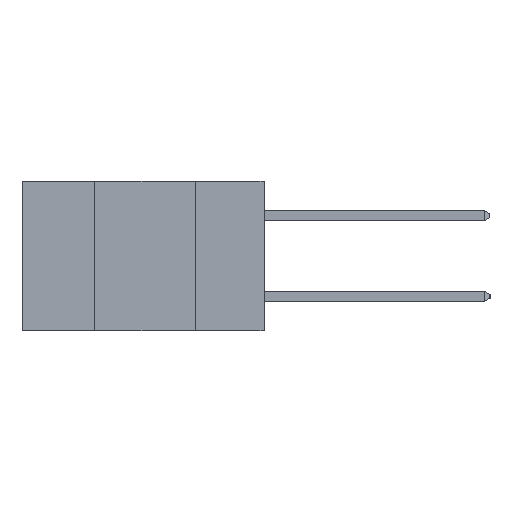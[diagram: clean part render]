
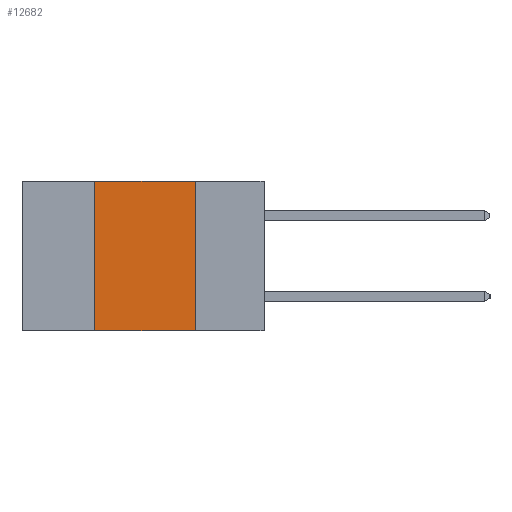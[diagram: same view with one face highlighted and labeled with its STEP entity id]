
A CAD part, left-side view. The second image highlights one B-rep face of the part: STEP entity #12682.
In plain terms, the highlighted planar face has unit normal (-1, 0, 0).
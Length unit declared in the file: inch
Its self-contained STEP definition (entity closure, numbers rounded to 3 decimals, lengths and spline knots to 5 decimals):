
#1041 = EDGE_CURVE ( 'NONE', #14348, #5909, #7604, .T. ) ;
#1482 = EDGE_LOOP ( 'NONE', ( #12746, #18399, #15497, #16934 ) ) ;
#1537 = VERTEX_POINT ( 'NONE', #18172 ) ;
#2102 = DIRECTION ( 'NONE',  ( 0., 0., -1. ) ) ;
#2430 = LINE ( 'NONE', #8013, #11968 ) ;
#3101 = DIRECTION ( 'NONE',  ( 0., -1., 0. ) ) ;
#3197 = DIRECTION ( 'NONE',  ( 0., -1., 0. ) ) ;
#4484 = VECTOR ( 'NONE', #3101, 39.37008 ) ;
#5244 = PLANE ( 'NONE',  #9983 ) ;
#5909 = VERTEX_POINT ( 'NONE', #8894 ) ;
#6665 = FACE_OUTER_BOUND ( 'NONE', #1482, .T. ) ;
#6901 = CARTESIAN_POINT ( 'NONE',  ( 0., 0.42, -0.37 ) ) ;
#7604 = LINE ( 'NONE', #6901, #19320 ) ;
#8013 = CARTESIAN_POINT ( 'NONE',  ( 0., 0.6, -0.37 ) ) ;
#8799 = DIRECTION ( 'NONE',  ( 0., 0., -1. ) ) ;
#8894 = CARTESIAN_POINT ( 'NONE',  ( 0., 0.42, 0. ) ) ;
#9983 = AXIS2_PLACEMENT_3D ( 'NONE', #10074, #11709, #2102 ) ;
#10074 = CARTESIAN_POINT ( 'NONE',  ( 0., 0.6, 0. ) ) ;
#10795 = CARTESIAN_POINT ( 'NONE',  ( 0., 0.42, -0.37 ) ) ;
#11117 = EDGE_CURVE ( 'NONE', #14348, #1537, #2430, .T. ) ;
#11612 = VECTOR ( 'NONE', #8799, 39.37008 ) ;
#11709 = DIRECTION ( 'NONE',  ( 1., 0., 0. ) ) ;
#11941 = DIRECTION ( 'NONE',  ( 0., 0., 1. ) ) ;
#11968 = VECTOR ( 'NONE', #3197, 39.37008 ) ;
#12682 = ADVANCED_FACE ( 'NONE', ( #6665 ), #5244, .F. ) ;
#12746 = ORIENTED_EDGE ( 'NONE', *, *, #14205, .F. ) ;
#13524 = LINE ( 'NONE', #19077, #4484 ) ;
#14205 = EDGE_CURVE ( 'NONE', #20488, #1537, #19538, .T. ) ;
#14348 = VERTEX_POINT ( 'NONE', #10795 ) ;
#15497 = ORIENTED_EDGE ( 'NONE', *, *, #1041, .F. ) ;
#16934 = ORIENTED_EDGE ( 'NONE', *, *, #11117, .T. ) ;
#17335 = CARTESIAN_POINT ( 'NONE',  ( 0., 0.17, 0. ) ) ;
#18172 = CARTESIAN_POINT ( 'NONE',  ( 0., 0.17, -0.37 ) ) ;
#18399 = ORIENTED_EDGE ( 'NONE', *, *, #19891, .F. ) ;
#19077 = CARTESIAN_POINT ( 'NONE',  ( 0., 0.6, 0. ) ) ;
#19320 = VECTOR ( 'NONE', #11941, 39.37008 ) ;
#19538 = LINE ( 'NONE', #19936, #11612 ) ;
#19891 = EDGE_CURVE ( 'NONE', #5909, #20488, #13524, .T. ) ;
#19936 = CARTESIAN_POINT ( 'NONE',  ( 0., 0.17, -0.37 ) ) ;
#20488 = VERTEX_POINT ( 'NONE', #17335 ) ;
